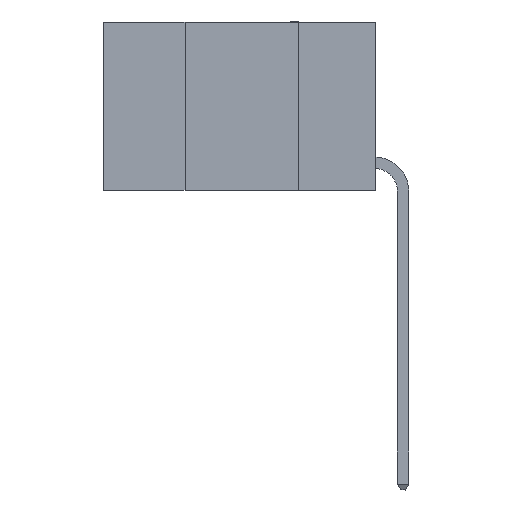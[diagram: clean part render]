
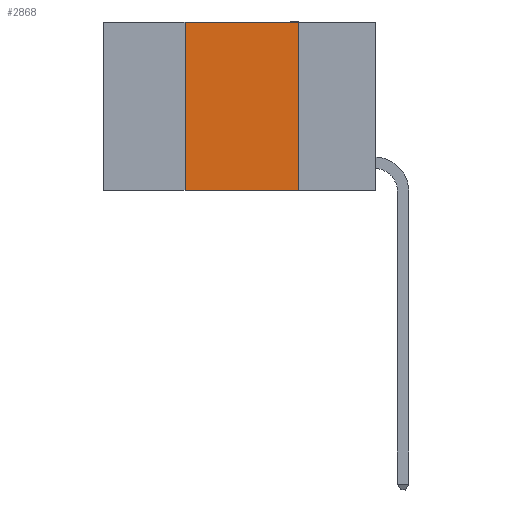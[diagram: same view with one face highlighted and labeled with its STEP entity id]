
A CAD part, left-side view. The second image highlights one B-rep face of the part: STEP entity #2868.
In plain terms, the highlighted planar face has unit normal (-1, 0, 0).
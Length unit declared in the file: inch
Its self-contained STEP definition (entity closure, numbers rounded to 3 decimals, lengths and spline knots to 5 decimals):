
#362 = VERTEX_POINT ( 'NONE', #9582 ) ;
#1192 = CARTESIAN_POINT ( 'NONE',  ( 0., 0.6, 0. ) ) ;
#2159 = ORIENTED_EDGE ( 'NONE', *, *, #18889, .T. ) ;
#2408 = CARTESIAN_POINT ( 'NONE',  ( 0., 0.17, 0. ) ) ;
#2868 = ADVANCED_FACE ( 'NONE', ( #15548 ), #19626, .F. ) ;
#3104 = DIRECTION ( 'NONE',  ( 0., -1., 0. ) ) ;
#3364 = DIRECTION ( 'NONE',  ( 0., 0., 1. ) ) ;
#3428 = EDGE_CURVE ( 'NONE', #21038, #11494, #22154, .T. ) ;
#3566 = VECTOR ( 'NONE', #14798, 39.37008 ) ;
#3749 = CARTESIAN_POINT ( 'NONE',  ( 0., 0.6, 0. ) ) ;
#6185 = CARTESIAN_POINT ( 'NONE',  ( 0., 0.17, 0. ) ) ;
#6316 = DIRECTION ( 'NONE',  ( 0., 0., -1. ) ) ;
#6712 = VERTEX_POINT ( 'NONE', #19672 ) ;
#6850 = LINE ( 'NONE', #16437, #14651 ) ;
#8878 = VECTOR ( 'NONE', #22022, 39.37008 ) ;
#8967 = CARTESIAN_POINT ( 'NONE',  ( 0., 0.17, -0.37 ) ) ;
#9582 = CARTESIAN_POINT ( 'NONE',  ( 0., 0.42, 0. ) ) ;
#11494 = VERTEX_POINT ( 'NONE', #8967 ) ;
#12134 = ORIENTED_EDGE ( 'NONE', *, *, #16211, .F. ) ;
#14651 = VECTOR ( 'NONE', #3364, 39.37008 ) ;
#14798 = DIRECTION ( 'NONE',  ( 0., -1., 0. ) ) ;
#15062 = VECTOR ( 'NONE', #3104, 39.37008 ) ;
#15548 = FACE_OUTER_BOUND ( 'NONE', #17840, .T. ) ;
#16211 = EDGE_CURVE ( 'NONE', #362, #21038, #22483, .T. ) ;
#16321 = CARTESIAN_POINT ( 'NONE',  ( 0., 0.6, -0.37 ) ) ;
#16437 = CARTESIAN_POINT ( 'NONE',  ( 0., 0.42, 0. ) ) ;
#17840 = EDGE_LOOP ( 'NONE', ( #18794, #12134, #18801, #2159 ) ) ;
#18794 = ORIENTED_EDGE ( 'NONE', *, *, #3428, .F. ) ;
#18801 = ORIENTED_EDGE ( 'NONE', *, *, #18952, .F. ) ;
#18889 = EDGE_CURVE ( 'NONE', #6712, #11494, #24245, .T. ) ;
#18952 = EDGE_CURVE ( 'NONE', #6712, #362, #6850, .T. ) ;
#19626 = PLANE ( 'NONE',  #22321 ) ;
#19672 = CARTESIAN_POINT ( 'NONE',  ( 0., 0.42, -0.37 ) ) ;
#21038 = VERTEX_POINT ( 'NONE', #6185 ) ;
#22022 = DIRECTION ( 'NONE',  ( 0., 0., -1. ) ) ;
#22154 = LINE ( 'NONE', #2408, #8878 ) ;
#22303 = DIRECTION ( 'NONE',  ( 1., 0., 0. ) ) ;
#22321 = AXIS2_PLACEMENT_3D ( 'NONE', #3749, #22303, #6316 ) ;
#22483 = LINE ( 'NONE', #1192, #3566 ) ;
#24245 = LINE ( 'NONE', #16321, #15062 ) ;
